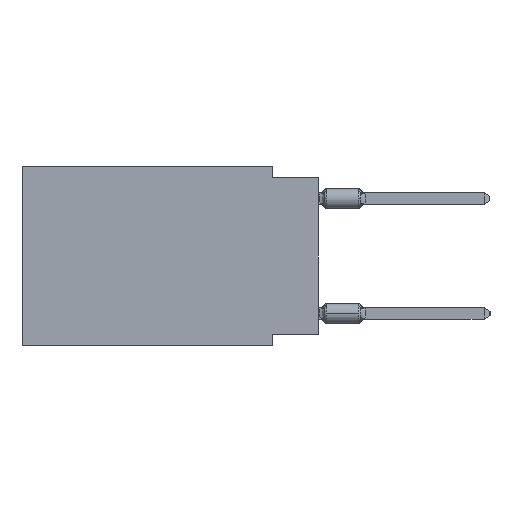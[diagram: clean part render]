
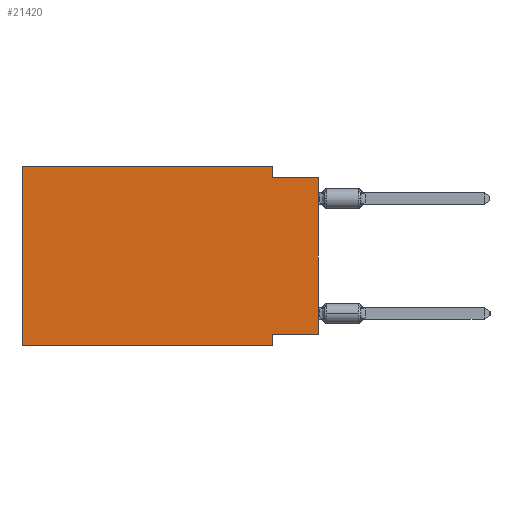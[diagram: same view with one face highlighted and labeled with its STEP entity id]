
A CAD part, left-side view. The second image highlights one B-rep face of the part: STEP entity #21420.
In plain terms, the highlighted planar face has unit normal (-1, 0, 0).
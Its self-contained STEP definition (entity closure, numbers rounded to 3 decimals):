
#217 = VECTOR ( 'NONE', #13950, 1000. ) ;
#1041 = EDGE_CURVE ( 'NONE', #1821, #21663, #34894, .T. ) ;
#1821 = VERTEX_POINT ( 'NONE', #28082 ) ;
#1845 = VECTOR ( 'NONE', #35525, 1000. ) ;
#3221 = ORIENTED_EDGE ( 'NONE', *, *, #29573, .F. ) ;
#3663 = DIRECTION ( 'NONE',  ( 0., 0., -1. ) ) ;
#4182 = CARTESIAN_POINT ( 'NONE',  ( 0., 16.383, -9.906 ) ) ;
#4548 = CARTESIAN_POINT ( 'NONE',  ( 0., 2.54, 0. ) ) ;
#4597 = EDGE_CURVE ( 'NONE', #41529, #11964, #20562, .T. ) ;
#7195 = VECTOR ( 'NONE', #14416, 1000. ) ;
#7224 = LINE ( 'NONE', #30489, #10097 ) ;
#7428 = DIRECTION ( 'NONE',  ( 0., 1., 0. ) ) ;
#7465 = CARTESIAN_POINT ( 'NONE',  ( 0., 16.383, 0. ) ) ;
#7621 = ORIENTED_EDGE ( 'NONE', *, *, #18001, .F. ) ;
#8002 = DIRECTION ( 'NONE',  ( 1., 0., 0. ) ) ;
#9457 = EDGE_CURVE ( 'NONE', #21663, #11964, #24365, .T. ) ;
#10097 = VECTOR ( 'NONE', #7428, 1000. ) ;
#11121 = CARTESIAN_POINT ( 'NONE',  ( 0., 2.54, -9.271 ) ) ;
#11964 = VERTEX_POINT ( 'NONE', #23485 ) ;
#12598 = LINE ( 'NONE', #33420, #35201 ) ;
#13950 = DIRECTION ( 'NONE',  ( 0., -1., 0. ) ) ;
#14416 = DIRECTION ( 'NONE',  ( 0., -1., 0. ) ) ;
#14603 = VECTOR ( 'NONE', #18043, 1000. ) ;
#15563 = LINE ( 'NONE', #34694, #1845 ) ;
#17752 = LINE ( 'NONE', #31263, #7195 ) ;
#18001 = EDGE_CURVE ( 'NONE', #32770, #23682, #31262, .T. ) ;
#18043 = DIRECTION ( 'NONE',  ( 0., 0., -1. ) ) ;
#20562 = LINE ( 'NONE', #27849, #36754 ) ;
#20901 = VECTOR ( 'NONE', #3663, 1000. ) ;
#21302 = CARTESIAN_POINT ( 'NONE',  ( 0., 2.54, -9.906 ) ) ;
#21420 = ADVANCED_FACE ( 'NONE', ( #34157 ), #41683, .F. ) ;
#21663 = VERTEX_POINT ( 'NONE', #32361 ) ;
#22526 = AXIS2_PLACEMENT_3D ( 'NONE', #24839, #8002, #41451 ) ;
#22768 = EDGE_CURVE ( 'NONE', #24806, #23682, #17752, .T. ) ;
#23485 = CARTESIAN_POINT ( 'NONE',  ( 0., 0., -0.635 ) ) ;
#23682 = VERTEX_POINT ( 'NONE', #30539 ) ;
#23887 = DIRECTION ( 'NONE',  ( 0., 0., 1. ) ) ;
#23891 = ORIENTED_EDGE ( 'NONE', *, *, #1041, .F. ) ;
#24066 = EDGE_CURVE ( 'NONE', #41529, #32770, #7224, .T. ) ;
#24365 = LINE ( 'NONE', #27241, #217 ) ;
#24806 = VERTEX_POINT ( 'NONE', #4182 ) ;
#24839 = CARTESIAN_POINT ( 'NONE',  ( 0., 16.383, 0. ) ) ;
#26773 = EDGE_LOOP ( 'NONE', ( #40306, #35613, #23891, #3221, #38899, #36839, #7621, #42142 ) ) ;
#26992 = DIRECTION ( 'NONE',  ( 0., 0., 1. ) ) ;
#27241 = CARTESIAN_POINT ( 'NONE',  ( 0., 0., -0.635 ) ) ;
#27849 = CARTESIAN_POINT ( 'NONE',  ( 0., 0., 0. ) ) ;
#28082 = CARTESIAN_POINT ( 'NONE',  ( 0., 2.54, 0. ) ) ;
#28602 = CARTESIAN_POINT ( 'NONE',  ( 0., 0., -9.271 ) ) ;
#29573 = EDGE_CURVE ( 'NONE', #35741, #1821, #15563, .T. ) ;
#30489 = CARTESIAN_POINT ( 'NONE',  ( 0., 0., -9.271 ) ) ;
#30539 = CARTESIAN_POINT ( 'NONE',  ( 0., 2.54, -9.906 ) ) ;
#31262 = LINE ( 'NONE', #21302, #20901 ) ;
#31263 = CARTESIAN_POINT ( 'NONE',  ( 0., 16.383, -9.906 ) ) ;
#32361 = CARTESIAN_POINT ( 'NONE',  ( 0., 2.54, -0.635 ) ) ;
#32770 = VERTEX_POINT ( 'NONE', #11121 ) ;
#33420 = CARTESIAN_POINT ( 'NONE',  ( 0., 16.383, 0. ) ) ;
#33448 = EDGE_CURVE ( 'NONE', #24806, #35741, #12598, .T. ) ;
#34157 = FACE_OUTER_BOUND ( 'NONE', #26773, .T. ) ;
#34694 = CARTESIAN_POINT ( 'NONE',  ( 0., 16.383, 0. ) ) ;
#34894 = LINE ( 'NONE', #4548, #14603 ) ;
#35201 = VECTOR ( 'NONE', #26992, 1000. ) ;
#35525 = DIRECTION ( 'NONE',  ( 0., -1., 0. ) ) ;
#35613 = ORIENTED_EDGE ( 'NONE', *, *, #9457, .F. ) ;
#35741 = VERTEX_POINT ( 'NONE', #7465 ) ;
#36754 = VECTOR ( 'NONE', #23887, 1000. ) ;
#36839 = ORIENTED_EDGE ( 'NONE', *, *, #22768, .T. ) ;
#38899 = ORIENTED_EDGE ( 'NONE', *, *, #33448, .F. ) ;
#40306 = ORIENTED_EDGE ( 'NONE', *, *, #4597, .T. ) ;
#41451 = DIRECTION ( 'NONE',  ( 0., 0., -1. ) ) ;
#41529 = VERTEX_POINT ( 'NONE', #28602 ) ;
#41683 = PLANE ( 'NONE',  #22526 ) ;
#42142 = ORIENTED_EDGE ( 'NONE', *, *, #24066, .F. ) ;
